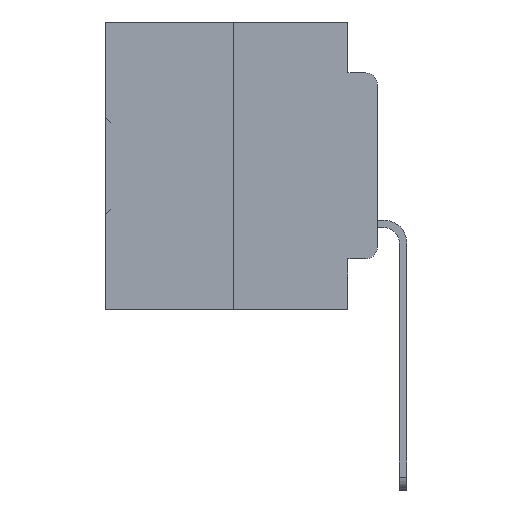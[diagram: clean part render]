
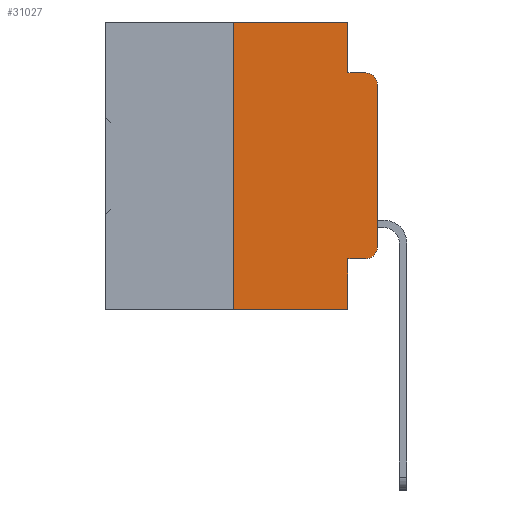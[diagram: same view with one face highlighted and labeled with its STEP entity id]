
A CAD part, left-side view. The second image highlights one B-rep face of the part: STEP entity #31027.
In plain terms, the highlighted planar face has unit normal (-1, 0, 0).
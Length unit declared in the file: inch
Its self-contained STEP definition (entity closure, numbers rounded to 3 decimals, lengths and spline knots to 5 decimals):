
#232 = DIRECTION ( 'NONE',  ( 0., 0., 1. ) ) ;
#404 = CARTESIAN_POINT ( 'NONE',  ( 0., 0.25, -0.5 ) ) ;
#753 = VERTEX_POINT ( 'NONE', #37174 ) ;
#1266 = VERTEX_POINT ( 'NONE', #8758 ) ;
#1422 = PLANE ( 'NONE',  #1532 ) ;
#1532 = AXIS2_PLACEMENT_3D ( 'NONE', #25376, #10599, #31409 ) ;
#2249 = ORIENTED_EDGE ( 'NONE', *, *, #22281, .T. ) ;
#3148 = CARTESIAN_POINT ( 'NONE',  ( 0., 0.051, -0.0885 ) ) ;
#3964 = EDGE_CURVE ( 'NONE', #6561, #1266, #21356, .T. ) ;
#4347 = CARTESIAN_POINT ( 'NONE',  ( 0., 0., 0. ) ) ;
#4582 = CIRCLE ( 'NONE', #38225, 0.02 ) ;
#4884 = EDGE_CURVE ( 'NONE', #10441, #753, #26442, .T. ) ;
#5051 = DIRECTION ( 'NONE',  ( 0., 0., -1. ) ) ;
#5428 = VECTOR ( 'NONE', #5051, 39.37008 ) ;
#5530 = VERTEX_POINT ( 'NONE', #7164 ) ;
#5652 = AXIS2_PLACEMENT_3D ( 'NONE', #25163, #7199, #28181 ) ;
#5692 = DIRECTION ( 'NONE',  ( -1., 0., 0. ) ) ;
#6561 = VERTEX_POINT ( 'NONE', #19367 ) ;
#6922 = DIRECTION ( 'NONE',  ( 0., -1., 0. ) ) ;
#7005 = FACE_OUTER_BOUND ( 'NONE', #13216, .T. ) ;
#7064 = CARTESIAN_POINT ( 'NONE',  ( 0., 0.051, 0. ) ) ;
#7164 = CARTESIAN_POINT ( 'NONE',  ( 0., 0.02, -0.0885 ) ) ;
#7199 = DIRECTION ( 'NONE',  ( -1., 0., 0. ) ) ;
#7833 = LINE ( 'NONE', #35988, #22854 ) ;
#8356 = LINE ( 'NONE', #3148, #15445 ) ;
#8522 = EDGE_CURVE ( 'NONE', #25528, #31749, #38249, .T. ) ;
#8758 = CARTESIAN_POINT ( 'NONE',  ( 0., 0.051, -0.0885 ) ) ;
#9492 = EDGE_CURVE ( 'NONE', #30709, #6561, #22126, .T. ) ;
#9977 = CARTESIAN_POINT ( 'NONE',  ( 0., 0.473, -0.5 ) ) ;
#10076 = EDGE_CURVE ( 'NONE', #753, #5530, #33137, .T. ) ;
#10289 = ORIENTED_EDGE ( 'NONE', *, *, #4884, .T. ) ;
#10441 = VERTEX_POINT ( 'NONE', #28854 ) ;
#10599 = DIRECTION ( 'NONE',  ( 1., 0., 0. ) ) ;
#12240 = VERTEX_POINT ( 'NONE', #404 ) ;
#13216 = EDGE_LOOP ( 'NONE', ( #10289, #22884, #31106, #23727, #19989, #13957, #15847, #25196, #33117, #2249 ) ) ;
#13957 = ORIENTED_EDGE ( 'NONE', *, *, #37320, .F. ) ;
#14057 = VERTEX_POINT ( 'NONE', #31839 ) ;
#15445 = VECTOR ( 'NONE', #30108, 39.37008 ) ;
#15847 = ORIENTED_EDGE ( 'NONE', *, *, #19307, .T. ) ;
#16319 = DIRECTION ( 'NONE',  ( 0., 0., 1. ) ) ;
#16405 = DIRECTION ( 'NONE',  ( 0., -1., 0. ) ) ;
#18302 = LINE ( 'NONE', #7064, #27138 ) ;
#18581 = CARTESIAN_POINT ( 'NONE',  ( 0., 0.473, 0. ) ) ;
#19307 = EDGE_CURVE ( 'NONE', #12240, #14057, #29851, .T. ) ;
#19367 = CARTESIAN_POINT ( 'NONE',  ( 0., 0.051, 0. ) ) ;
#19989 = ORIENTED_EDGE ( 'NONE', *, *, #9492, .F. ) ;
#21356 = LINE ( 'NONE', #23008, #5428 ) ;
#22126 = LINE ( 'NONE', #18581, #36812 ) ;
#22281 = EDGE_CURVE ( 'NONE', #31749, #10441, #4582, .T. ) ;
#22854 = VECTOR ( 'NONE', #232, 39.37008 ) ;
#22884 = ORIENTED_EDGE ( 'NONE', *, *, #10076, .T. ) ;
#23008 = CARTESIAN_POINT ( 'NONE',  ( 0., 0.051, 0. ) ) ;
#23624 = VECTOR ( 'NONE', #16405, 39.37008 ) ;
#23643 = CARTESIAN_POINT ( 'NONE',  ( 0., 0.02, -0.3915 ) ) ;
#23727 = ORIENTED_EDGE ( 'NONE', *, *, #3964, .F. ) ;
#24558 = DIRECTION ( 'NONE',  ( 0., -1., 0. ) ) ;
#25163 = CARTESIAN_POINT ( 'NONE',  ( 0., 0.02, -0.1085 ) ) ;
#25196 = ORIENTED_EDGE ( 'NONE', *, *, #26620, .F. ) ;
#25376 = CARTESIAN_POINT ( 'NONE',  ( 0., 0.473, 0. ) ) ;
#25528 = VERTEX_POINT ( 'NONE', #31724 ) ;
#26442 = LINE ( 'NONE', #4347, #27362 ) ;
#26620 = EDGE_CURVE ( 'NONE', #25528, #14057, #18302, .T. ) ;
#26639 = DIRECTION ( 'NONE',  ( 0., 0., -1. ) ) ;
#27138 = VECTOR ( 'NONE', #28029, 39.37008 ) ;
#27362 = VECTOR ( 'NONE', #16319, 39.37008 ) ;
#28029 = DIRECTION ( 'NONE',  ( 0., 0., -1. ) ) ;
#28181 = DIRECTION ( 'NONE',  ( 0., 0., -1. ) ) ;
#28854 = CARTESIAN_POINT ( 'NONE',  ( 0., 0., -0.3915 ) ) ;
#29851 = LINE ( 'NONE', #9977, #36626 ) ;
#30108 = DIRECTION ( 'NONE',  ( 0., -1., 0. ) ) ;
#30709 = VERTEX_POINT ( 'NONE', #38620 ) ;
#31027 = ADVANCED_FACE ( 'NONE', ( #7005 ), #1422, .F. ) ;
#31106 = ORIENTED_EDGE ( 'NONE', *, *, #36652, .F. ) ;
#31409 = DIRECTION ( 'NONE',  ( 0., 0., -1. ) ) ;
#31599 = CARTESIAN_POINT ( 'NONE',  ( 0., 0.02, -0.4115 ) ) ;
#31724 = CARTESIAN_POINT ( 'NONE',  ( 0., 0.051, -0.4115 ) ) ;
#31749 = VERTEX_POINT ( 'NONE', #31599 ) ;
#31839 = CARTESIAN_POINT ( 'NONE',  ( 0., 0.051, -0.5 ) ) ;
#33117 = ORIENTED_EDGE ( 'NONE', *, *, #8522, .T. ) ;
#33137 = CIRCLE ( 'NONE', #5652, 0.02 ) ;
#34087 = CARTESIAN_POINT ( 'NONE',  ( 0., 0.051, -0.4115 ) ) ;
#35988 = CARTESIAN_POINT ( 'NONE',  ( 0., 0.25, 0. ) ) ;
#36626 = VECTOR ( 'NONE', #6922, 39.37008 ) ;
#36652 = EDGE_CURVE ( 'NONE', #1266, #5530, #8356, .T. ) ;
#36812 = VECTOR ( 'NONE', #24558, 39.37008 ) ;
#37174 = CARTESIAN_POINT ( 'NONE',  ( 0., 0., -0.1085 ) ) ;
#37320 = EDGE_CURVE ( 'NONE', #12240, #30709, #7833, .T. ) ;
#38225 = AXIS2_PLACEMENT_3D ( 'NONE', #23643, #5692, #26639 ) ;
#38249 = LINE ( 'NONE', #34087, #23624 ) ;
#38620 = CARTESIAN_POINT ( 'NONE',  ( 0., 0.25, 0. ) ) ;
